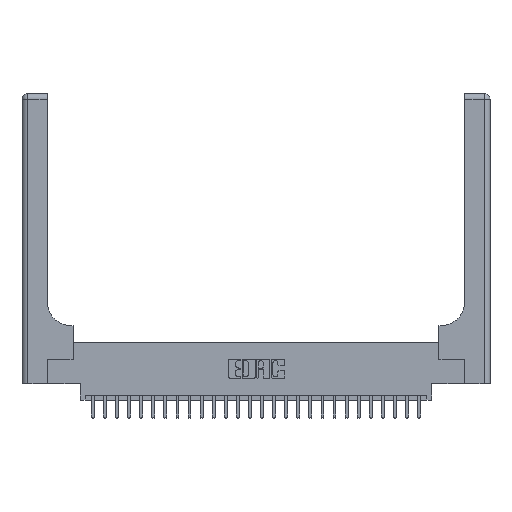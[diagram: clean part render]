
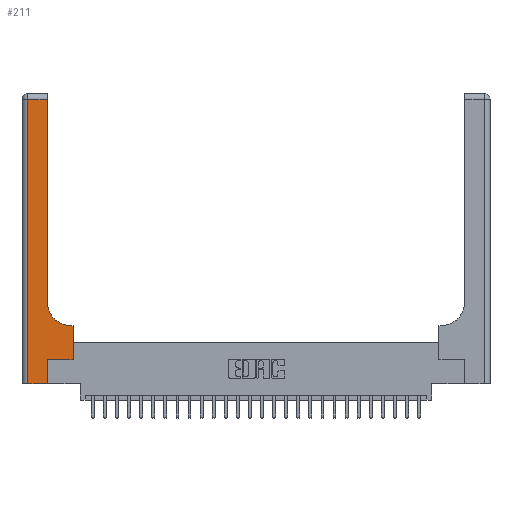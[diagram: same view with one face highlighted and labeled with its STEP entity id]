
A CAD part, top view. The second image highlights one B-rep face of the part: STEP entity #211.
In plain terms, the highlighted planar face has unit normal (0, 0, 1).
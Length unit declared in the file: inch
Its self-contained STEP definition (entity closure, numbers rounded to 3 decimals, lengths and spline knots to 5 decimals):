
#211 = ADVANCED_FACE ( 'NONE', ( #5477 ), #16039, .F. ) ;
#397 = LINE ( 'NONE', #12047, #10519 ) ;
#775 = CARTESIAN_POINT ( 'NONE',  ( 0.06, 3., 0.37 ) ) ;
#2091 = DIRECTION ( 'NONE',  ( 0., 1., 0. ) ) ;
#2631 = VERTEX_POINT ( 'NONE', #11009 ) ;
#2810 = ORIENTED_EDGE ( 'NONE', *, *, #3084, .T. ) ;
#2822 = DIRECTION ( 'NONE',  ( 0., -1., 0. ) ) ;
#3084 = EDGE_CURVE ( 'NONE', #20558, #17532, #25492, .T. ) ;
#3409 = DIRECTION ( 'NONE',  ( 1., 0., 0. ) ) ;
#3560 = CARTESIAN_POINT ( 'NONE',  ( 0., 0., 0.37 ) ) ;
#3977 = DIRECTION ( 'NONE',  ( -1., 0., 0. ) ) ;
#4655 = CARTESIAN_POINT ( 'NONE',  ( 0.265, 0., 0.37 ) ) ;
#4734 = ORIENTED_EDGE ( 'NONE', *, *, #5667, .T. ) ;
#5477 = FACE_OUTER_BOUND ( 'NONE', #10604, .T. ) ;
#5667 = EDGE_CURVE ( 'NONE', #11037, #17110, #7290, .T. ) ;
#6626 = VECTOR ( 'NONE', #2822, 39.37008 ) ;
#6923 = ORIENTED_EDGE ( 'NONE', *, *, #20677, .T. ) ;
#7126 = CARTESIAN_POINT ( 'NONE',  ( 0.51, 0.85, 0.37 ) ) ;
#7290 = LINE ( 'NONE', #10576, #17881 ) ;
#7523 = ORIENTED_EDGE ( 'NONE', *, *, #9702, .T. ) ;
#9140 = DIRECTION ( 'NONE',  ( 1., 0., 0. ) ) ;
#9410 = LINE ( 'NONE', #25413, #18720 ) ;
#9702 = EDGE_CURVE ( 'NONE', #2631, #20638, #25049, .T. ) ;
#9972 = CARTESIAN_POINT ( 'NONE',  ( 0.51, 0.6, 0.37 ) ) ;
#10519 = VECTOR ( 'NONE', #14020, 39.37008 ) ;
#10576 = CARTESIAN_POINT ( 'NONE',  ( 0.528, 0.25, 0.37 ) ) ;
#10604 = EDGE_LOOP ( 'NONE', ( #16238, #7523, #6923, #2810, #19348, #24460, #4734, #15958, #21786 ) ) ;
#10697 = EDGE_CURVE ( 'NONE', #14693, #2631, #9410, .T. ) ;
#10743 = CARTESIAN_POINT ( 'NONE',  ( 0.528, 0.25, 0.37 ) ) ;
#11009 = CARTESIAN_POINT ( 'NONE',  ( 0.26, 2.94, 0.37 ) ) ;
#11037 = VERTEX_POINT ( 'NONE', #10743 ) ;
#11200 = CARTESIAN_POINT ( 'NONE',  ( 0.26, 0.85, 0.37 ) ) ;
#11657 = VERTEX_POINT ( 'NONE', #14257 ) ;
#12047 = CARTESIAN_POINT ( 'NONE',  ( 0.265, 0.25, 0.37 ) ) ;
#12258 = VERTEX_POINT ( 'NONE', #9972 ) ;
#12656 = VECTOR ( 'NONE', #2091, 39.37008 ) ;
#13376 = CARTESIAN_POINT ( 'NONE',  ( 0.528, 0.6, 0.37 ) ) ;
#13493 = EDGE_CURVE ( 'NONE', #17532, #11657, #23117, .T. ) ;
#14020 = DIRECTION ( 'NONE',  ( 1., 0., 0. ) ) ;
#14257 = CARTESIAN_POINT ( 'NONE',  ( 0.265, 0.25, 0.37 ) ) ;
#14595 = VECTOR ( 'NONE', #3409, 39.37008 ) ;
#14693 = VERTEX_POINT ( 'NONE', #11200 ) ;
#14845 = LINE ( 'NONE', #21075, #24576 ) ;
#15780 = DIRECTION ( 'NONE',  ( 0., 1., 0. ) ) ;
#15860 = AXIS2_PLACEMENT_3D ( 'NONE', #15971, #15916, #15862 ) ;
#15862 = DIRECTION ( 'NONE',  ( -1., 0., 0. ) ) ;
#15916 = DIRECTION ( 'NONE',  ( 0., 0., -1. ) ) ;
#15922 = CARTESIAN_POINT ( 'NONE',  ( 0., 2.94, 0.37 ) ) ;
#15958 = ORIENTED_EDGE ( 'NONE', *, *, #22692, .T. ) ;
#15971 = CARTESIAN_POINT ( 'NONE',  ( 0., 3., 0.37 ) ) ;
#16039 = PLANE ( 'NONE',  #15860 ) ;
#16238 = ORIENTED_EDGE ( 'NONE', *, *, #10697, .T. ) ;
#16646 = CARTESIAN_POINT ( 'NONE',  ( 0.06, 2.94, 0.37 ) ) ;
#17110 = VERTEX_POINT ( 'NONE', #13376 ) ;
#17123 = AXIS2_PLACEMENT_3D ( 'NONE', #7126, #20970, #9140 ) ;
#17200 = LINE ( 'NONE', #775, #6626 ) ;
#17532 = VERTEX_POINT ( 'NONE', #4655 ) ;
#17881 = VECTOR ( 'NONE', #24296, 39.37008 ) ;
#18395 = CARTESIAN_POINT ( 'NONE',  ( 0.06, 0., 0.37 ) ) ;
#18720 = VECTOR ( 'NONE', #15780, 39.37008 ) ;
#18971 = EDGE_CURVE ( 'NONE', #12258, #14693, #19446, .T. ) ;
#19348 = ORIENTED_EDGE ( 'NONE', *, *, #13493, .T. ) ;
#19446 = CIRCLE ( 'NONE', #17123, 0.25 ) ;
#20558 = VERTEX_POINT ( 'NONE', #18395 ) ;
#20638 = VERTEX_POINT ( 'NONE', #16646 ) ;
#20677 = EDGE_CURVE ( 'NONE', #20638, #20558, #17200, .T. ) ;
#20970 = DIRECTION ( 'NONE',  ( 0., 0., -1. ) ) ;
#21075 = CARTESIAN_POINT ( 'NONE',  ( 0.26, 0.6, 0.37 ) ) ;
#21786 = ORIENTED_EDGE ( 'NONE', *, *, #18971, .T. ) ;
#22408 = EDGE_CURVE ( 'NONE', #11657, #11037, #397, .T. ) ;
#22692 = EDGE_CURVE ( 'NONE', #17110, #12258, #14845, .T. ) ;
#23018 = DIRECTION ( 'NONE',  ( -1., 0., 0. ) ) ;
#23117 = LINE ( 'NONE', #24018, #12656 ) ;
#23905 = VECTOR ( 'NONE', #3977, 39.37008 ) ;
#24018 = CARTESIAN_POINT ( 'NONE',  ( 0.265, 0., 0.37 ) ) ;
#24296 = DIRECTION ( 'NONE',  ( 0., 1., 0. ) ) ;
#24460 = ORIENTED_EDGE ( 'NONE', *, *, #22408, .T. ) ;
#24576 = VECTOR ( 'NONE', #23018, 39.37008 ) ;
#25049 = LINE ( 'NONE', #15922, #23905 ) ;
#25413 = CARTESIAN_POINT ( 'NONE',  ( 0.26, 3., 0.37 ) ) ;
#25492 = LINE ( 'NONE', #3560, #14595 ) ;
